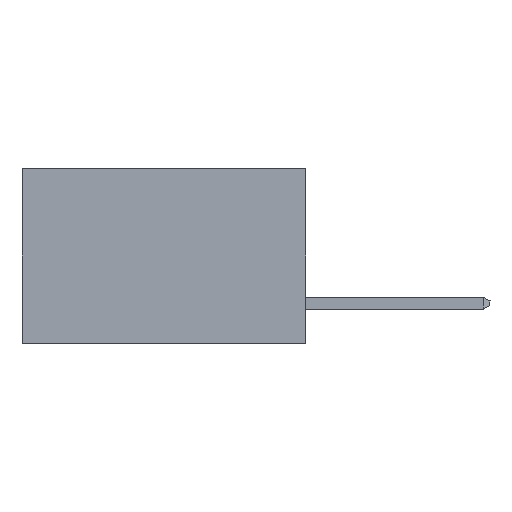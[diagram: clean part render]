
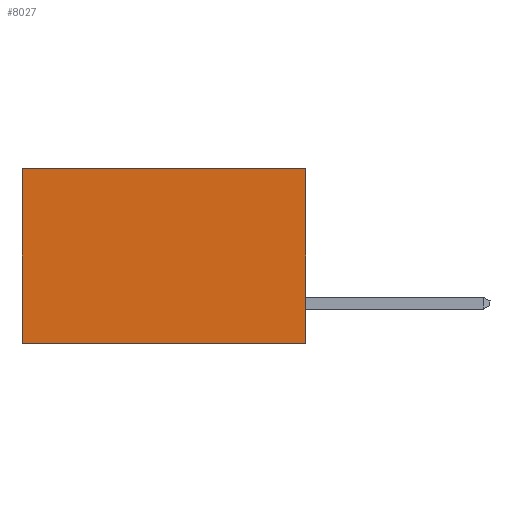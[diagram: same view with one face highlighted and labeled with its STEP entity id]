
A CAD part, left-side view. The second image highlights one B-rep face of the part: STEP entity #8027.
In plain terms, the highlighted planar face has unit normal (-1, 0, 0).
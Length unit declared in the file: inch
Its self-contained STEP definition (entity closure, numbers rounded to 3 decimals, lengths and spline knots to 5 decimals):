
#115 = EDGE_CURVE ( 'NONE', #859, #4088, #3773, .T. ) ;
#638 = LINE ( 'NONE', #2353, #9558 ) ;
#848 = CARTESIAN_POINT ( 'NONE',  ( 0.298, 0., -0.37 ) ) ;
#859 = VERTEX_POINT ( 'NONE', #6846 ) ;
#1766 = ORIENTED_EDGE ( 'NONE', *, *, #6182, .F. ) ;
#1817 = LINE ( 'NONE', #11795, #11849 ) ;
#2308 = PLANE ( 'NONE',  #2375 ) ;
#2353 = CARTESIAN_POINT ( 'NONE',  ( 0.298, 0., 0. ) ) ;
#2375 = AXIS2_PLACEMENT_3D ( 'NONE', #12940, #22977, #14711 ) ;
#3773 = LINE ( 'NONE', #8234, #14354 ) ;
#4088 = VERTEX_POINT ( 'NONE', #20208 ) ;
#4516 = EDGE_CURVE ( 'NONE', #9832, #5274, #1817, .T. ) ;
#5274 = VERTEX_POINT ( 'NONE', #12665 ) ;
#5382 = ORIENTED_EDGE ( 'NONE', *, *, #4516, .T. ) ;
#5606 = EDGE_LOOP ( 'NONE', ( #5382, #1766, #6798, #10441 ) ) ;
#5613 = LINE ( 'NONE', #848, #9253 ) ;
#5916 = EDGE_CURVE ( 'NONE', #859, #9832, #638, .T. ) ;
#6182 = EDGE_CURVE ( 'NONE', #4088, #5274, #5613, .T. ) ;
#6339 = DIRECTION ( 'NONE',  ( 0., 0., -1. ) ) ;
#6798 = ORIENTED_EDGE ( 'NONE', *, *, #115, .F. ) ;
#6846 = CARTESIAN_POINT ( 'NONE',  ( 0.298, 0., 0. ) ) ;
#8027 = ADVANCED_FACE ( 'NONE', ( #10843 ), #2308, .F. ) ;
#8234 = CARTESIAN_POINT ( 'NONE',  ( 0.298, 0., 0. ) ) ;
#9253 = VECTOR ( 'NONE', #22152, 39.37008 ) ;
#9558 = VECTOR ( 'NONE', #14759, 39.37008 ) ;
#9832 = VERTEX_POINT ( 'NONE', #19888 ) ;
#10441 = ORIENTED_EDGE ( 'NONE', *, *, #5916, .T. ) ;
#10843 = FACE_OUTER_BOUND ( 'NONE', #5606, .T. ) ;
#11795 = CARTESIAN_POINT ( 'NONE',  ( 0.298, 0.6, 0. ) ) ;
#11849 = VECTOR ( 'NONE', #20121, 39.37008 ) ;
#12665 = CARTESIAN_POINT ( 'NONE',  ( 0.298, 0.6, -0.37 ) ) ;
#12940 = CARTESIAN_POINT ( 'NONE',  ( 0.298, 0., 0. ) ) ;
#14354 = VECTOR ( 'NONE', #6339, 39.37008 ) ;
#14711 = DIRECTION ( 'NONE',  ( 0., 0., -1. ) ) ;
#14759 = DIRECTION ( 'NONE',  ( 0., 1., 0. ) ) ;
#19888 = CARTESIAN_POINT ( 'NONE',  ( 0.298, 0.6, 0. ) ) ;
#20121 = DIRECTION ( 'NONE',  ( 0., 0., -1. ) ) ;
#20208 = CARTESIAN_POINT ( 'NONE',  ( 0.298, 0., -0.37 ) ) ;
#22152 = DIRECTION ( 'NONE',  ( 0., 1., 0. ) ) ;
#22977 = DIRECTION ( 'NONE',  ( 1., 0., 0. ) ) ;
